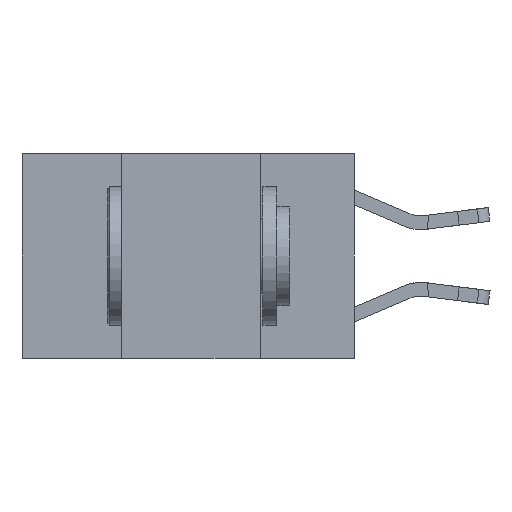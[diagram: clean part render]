
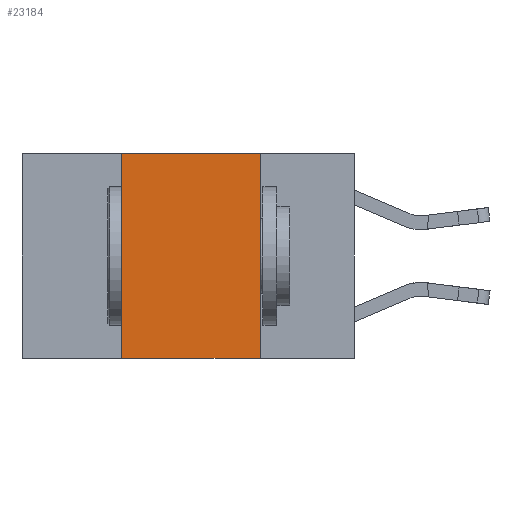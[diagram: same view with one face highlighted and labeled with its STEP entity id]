
A CAD part, left-side view. The second image highlights one B-rep face of the part: STEP entity #23184.
In plain terms, the highlighted planar face has unit normal (-1, 0, 0).
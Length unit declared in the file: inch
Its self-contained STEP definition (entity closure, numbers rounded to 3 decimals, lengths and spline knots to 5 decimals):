
#35 = LINE ( 'NONE', #6318, #9917 ) ;
#128 = ORIENTED_EDGE ( 'NONE', *, *, #21323, .F. ) ;
#596 = EDGE_LOOP ( 'NONE', ( #23243, #14061, #128, #21766 ) ) ;
#2310 = EDGE_CURVE ( 'NONE', #15110, #16453, #7992, .T. ) ;
#2464 = PLANE ( 'NONE',  #11463 ) ;
#2505 = CARTESIAN_POINT ( 'NONE',  ( 0., 0.17, -0.37 ) ) ;
#2770 = VECTOR ( 'NONE', #7118, 39.37008 ) ;
#2971 = CARTESIAN_POINT ( 'NONE',  ( 0., 0.6, 0. ) ) ;
#3377 = CARTESIAN_POINT ( 'NONE',  ( 0., 0.42, 0. ) ) ;
#4342 = DIRECTION ( 'NONE',  ( 0., -1., 0. ) ) ;
#4400 = VERTEX_POINT ( 'NONE', #3377 ) ;
#6318 = CARTESIAN_POINT ( 'NONE',  ( 0., 0.6, -0.37 ) ) ;
#7118 = DIRECTION ( 'NONE',  ( 0., 0., -1. ) ) ;
#7173 = FACE_OUTER_BOUND ( 'NONE', #596, .T. ) ;
#7992 = LINE ( 'NONE', #12971, #2770 ) ;
#8400 = DIRECTION ( 'NONE',  ( 1., 0., 0. ) ) ;
#8782 = CARTESIAN_POINT ( 'NONE',  ( 0., 0.42, -0.37 ) ) ;
#9049 = EDGE_CURVE ( 'NONE', #10990, #16453, #35, .T. ) ;
#9229 = EDGE_CURVE ( 'NONE', #4400, #15110, #12076, .T. ) ;
#9917 = VECTOR ( 'NONE', #4342, 39.37008 ) ;
#10589 = CARTESIAN_POINT ( 'NONE',  ( 0., 0.42, 0. ) ) ;
#10990 = VERTEX_POINT ( 'NONE', #8782 ) ;
#11463 = AXIS2_PLACEMENT_3D ( 'NONE', #20290, #8400, #22209 ) ;
#12076 = LINE ( 'NONE', #2971, #16826 ) ;
#12595 = DIRECTION ( 'NONE',  ( 0., 0., 1. ) ) ;
#12780 = DIRECTION ( 'NONE',  ( 0., -1., 0. ) ) ;
#12971 = CARTESIAN_POINT ( 'NONE',  ( 0., 0.17, 0. ) ) ;
#13461 = CARTESIAN_POINT ( 'NONE',  ( 0., 0.17, 0. ) ) ;
#14061 = ORIENTED_EDGE ( 'NONE', *, *, #9229, .F. ) ;
#15110 = VERTEX_POINT ( 'NONE', #13461 ) ;
#16453 = VERTEX_POINT ( 'NONE', #2505 ) ;
#16826 = VECTOR ( 'NONE', #12780, 39.37008 ) ;
#18144 = VECTOR ( 'NONE', #12595, 39.37008 ) ;
#18774 = LINE ( 'NONE', #10589, #18144 ) ;
#20290 = CARTESIAN_POINT ( 'NONE',  ( 0., 0.6, 0. ) ) ;
#21323 = EDGE_CURVE ( 'NONE', #10990, #4400, #18774, .T. ) ;
#21766 = ORIENTED_EDGE ( 'NONE', *, *, #9049, .T. ) ;
#22209 = DIRECTION ( 'NONE',  ( 0., 0., -1. ) ) ;
#23184 = ADVANCED_FACE ( 'NONE', ( #7173 ), #2464, .F. ) ;
#23243 = ORIENTED_EDGE ( 'NONE', *, *, #2310, .F. ) ;
